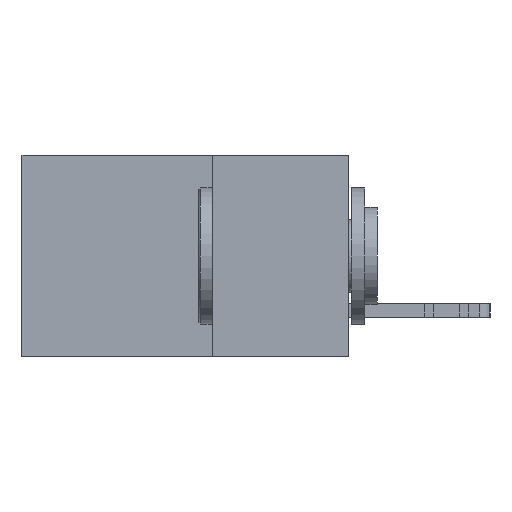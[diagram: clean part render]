
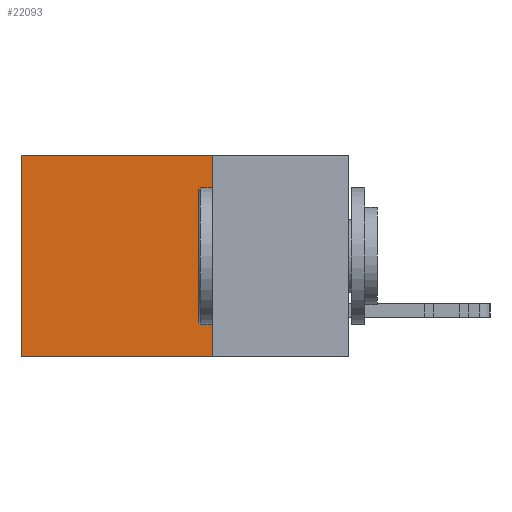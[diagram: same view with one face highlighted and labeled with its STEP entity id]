
A CAD part, left-side view. The second image highlights one B-rep face of the part: STEP entity #22093.
In plain terms, the highlighted planar face has unit normal (-1, 0, 0).
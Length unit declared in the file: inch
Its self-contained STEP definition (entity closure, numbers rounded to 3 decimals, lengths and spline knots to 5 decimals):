
#87 = CARTESIAN_POINT ( 'NONE',  ( 0.298, 0.25, -0.37 ) ) ;
#2613 = LINE ( 'NONE', #22587, #8478 ) ;
#3183 = DIRECTION ( 'NONE',  ( 1., 0., 0. ) ) ;
#3190 = ORIENTED_EDGE ( 'NONE', *, *, #11221, .T. ) ;
#3852 = VERTEX_POINT ( 'NONE', #30680 ) ;
#4488 = VECTOR ( 'NONE', #27738, 39.37008 ) ;
#5010 = DIRECTION ( 'NONE',  ( 0., 1., 0. ) ) ;
#6269 = EDGE_CURVE ( 'NONE', #18454, #3852, #31106, .T. ) ;
#6502 = LINE ( 'NONE', #16645, #32320 ) ;
#8478 = VECTOR ( 'NONE', #10063, 39.37008 ) ;
#8874 = ORIENTED_EDGE ( 'NONE', *, *, #6269, .T. ) ;
#9273 = DIRECTION ( 'NONE',  ( 0., 0., -1. ) ) ;
#10063 = DIRECTION ( 'NONE',  ( 0., 0., -1. ) ) ;
#11221 = EDGE_CURVE ( 'NONE', #3852, #28081, #2613, .T. ) ;
#11842 = VERTEX_POINT ( 'NONE', #27245 ) ;
#13833 = EDGE_CURVE ( 'NONE', #11842, #28081, #31913, .T. ) ;
#14277 = ORIENTED_EDGE ( 'NONE', *, *, #27725, .F. ) ;
#14560 = CARTESIAN_POINT ( 'NONE',  ( 0.298, 0.25, 0. ) ) ;
#16645 = CARTESIAN_POINT ( 'NONE',  ( 0.298, 0.25, 0. ) ) ;
#17511 = ORIENTED_EDGE ( 'NONE', *, *, #13833, .F. ) ;
#18180 = PLANE ( 'NONE',  #23152 ) ;
#18454 = VERTEX_POINT ( 'NONE', #14560 ) ;
#20568 = CARTESIAN_POINT ( 'NONE',  ( 0.298, 0.6, -0.37 ) ) ;
#20698 = DIRECTION ( 'NONE',  ( 0., 0., -1. ) ) ;
#22093 = ADVANCED_FACE ( 'NONE', ( #24972 ), #18180, .F. ) ;
#22587 = CARTESIAN_POINT ( 'NONE',  ( 0.298, 0.6, 0. ) ) ;
#23108 = CARTESIAN_POINT ( 'NONE',  ( 0.298, 0.25, 0. ) ) ;
#23152 = AXIS2_PLACEMENT_3D ( 'NONE', #23108, #3183, #20698 ) ;
#24972 = FACE_OUTER_BOUND ( 'NONE', #27017, .T. ) ;
#25277 = VECTOR ( 'NONE', #5010, 39.37008 ) ;
#27017 = EDGE_LOOP ( 'NONE', ( #3190, #17511, #14277, #8874 ) ) ;
#27245 = CARTESIAN_POINT ( 'NONE',  ( 0.298, 0.25, -0.37 ) ) ;
#27725 = EDGE_CURVE ( 'NONE', #18454, #11842, #6502, .T. ) ;
#27738 = DIRECTION ( 'NONE',  ( 0., 1., 0. ) ) ;
#28081 = VERTEX_POINT ( 'NONE', #20568 ) ;
#30229 = CARTESIAN_POINT ( 'NONE',  ( 0.298, 0.25, 0. ) ) ;
#30680 = CARTESIAN_POINT ( 'NONE',  ( 0.298, 0.6, 0. ) ) ;
#31106 = LINE ( 'NONE', #30229, #4488 ) ;
#31913 = LINE ( 'NONE', #87, #25277 ) ;
#32320 = VECTOR ( 'NONE', #9273, 39.37008 ) ;
